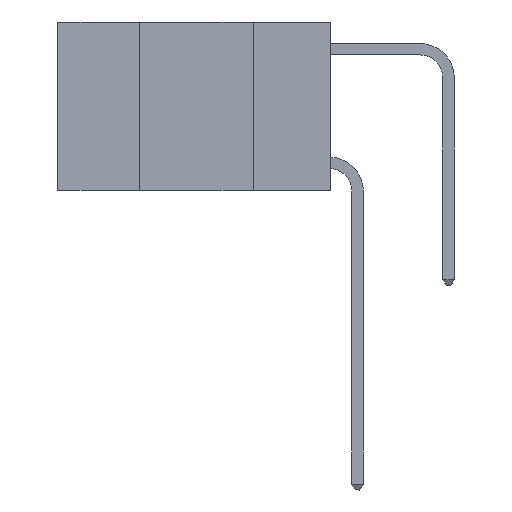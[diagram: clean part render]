
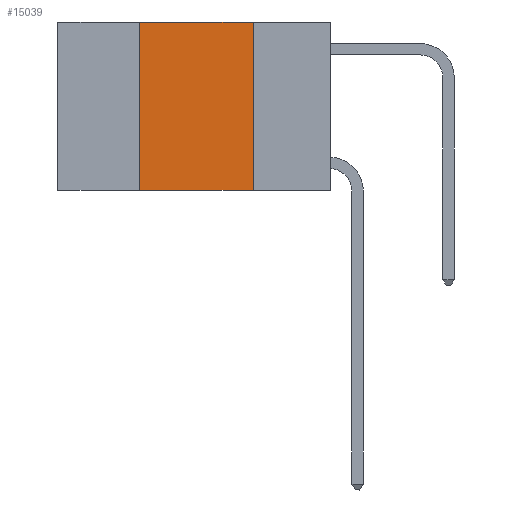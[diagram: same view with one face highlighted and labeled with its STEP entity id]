
A CAD part, left-side view. The second image highlights one B-rep face of the part: STEP entity #15039.
In plain terms, the highlighted planar face has unit normal (-1, 0, 0).
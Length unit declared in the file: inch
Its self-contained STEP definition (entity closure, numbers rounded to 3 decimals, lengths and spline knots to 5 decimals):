
#117 = CARTESIAN_POINT ( 'NONE',  ( 0., 0.6, -0.37 ) ) ;
#286 = CARTESIAN_POINT ( 'NONE',  ( 0., 0.42, -0.37 ) ) ;
#616 = EDGE_CURVE ( 'NONE', #9785, #4016, #8917, .T. ) ;
#1211 = CARTESIAN_POINT ( 'NONE',  ( 0., 0.17, -0.37 ) ) ;
#2241 = VERTEX_POINT ( 'NONE', #20521 ) ;
#2930 = DIRECTION ( 'NONE',  ( 0., -1., 0. ) ) ;
#3388 = EDGE_LOOP ( 'NONE', ( #19042, #6240, #18567, #5735 ) ) ;
#4016 = VERTEX_POINT ( 'NONE', #13619 ) ;
#5147 = EDGE_CURVE ( 'NONE', #2241, #17188, #17784, .T. ) ;
#5735 = ORIENTED_EDGE ( 'NONE', *, *, #8438, .T. ) ;
#5757 = EDGE_CURVE ( 'NONE', #4016, #2241, #12274, .T. ) ;
#5830 = PLANE ( 'NONE',  #10017 ) ;
#6240 = ORIENTED_EDGE ( 'NONE', *, *, #5757, .F. ) ;
#6575 = CARTESIAN_POINT ( 'NONE',  ( 0., 0.17, 0. ) ) ;
#6811 = DIRECTION ( 'NONE',  ( 0., -1., 0. ) ) ;
#8438 = EDGE_CURVE ( 'NONE', #9785, #17188, #16160, .T. ) ;
#8917 = LINE ( 'NONE', #17362, #9412 ) ;
#9076 = CARTESIAN_POINT ( 'NONE',  ( 0., 0.6, 0. ) ) ;
#9412 = VECTOR ( 'NONE', #13385, 39.37008 ) ;
#9785 = VERTEX_POINT ( 'NONE', #286 ) ;
#9913 = FACE_OUTER_BOUND ( 'NONE', #3388, .T. ) ;
#10017 = AXIS2_PLACEMENT_3D ( 'NONE', #9076, #20255, #10711 ) ;
#10711 = DIRECTION ( 'NONE',  ( 0., 0., -1. ) ) ;
#11154 = CARTESIAN_POINT ( 'NONE',  ( 0., 0.6, 0. ) ) ;
#12274 = LINE ( 'NONE', #11154, #19754 ) ;
#13070 = DIRECTION ( 'NONE',  ( 0., 0., -1. ) ) ;
#13385 = DIRECTION ( 'NONE',  ( 0., 0., 1. ) ) ;
#13534 = VECTOR ( 'NONE', #13070, 39.37008 ) ;
#13619 = CARTESIAN_POINT ( 'NONE',  ( 0., 0.42, 0. ) ) ;
#15039 = ADVANCED_FACE ( 'NONE', ( #9913 ), #5830, .F. ) ;
#15144 = VECTOR ( 'NONE', #6811, 39.37008 ) ;
#16160 = LINE ( 'NONE', #117, #15144 ) ;
#17188 = VERTEX_POINT ( 'NONE', #1211 ) ;
#17362 = CARTESIAN_POINT ( 'NONE',  ( 0., 0.42, 0. ) ) ;
#17784 = LINE ( 'NONE', #6575, #13534 ) ;
#18567 = ORIENTED_EDGE ( 'NONE', *, *, #616, .F. ) ;
#19042 = ORIENTED_EDGE ( 'NONE', *, *, #5147, .F. ) ;
#19754 = VECTOR ( 'NONE', #2930, 39.37008 ) ;
#20255 = DIRECTION ( 'NONE',  ( 1., 0., 0. ) ) ;
#20521 = CARTESIAN_POINT ( 'NONE',  ( 0., 0.17, 0. ) ) ;
